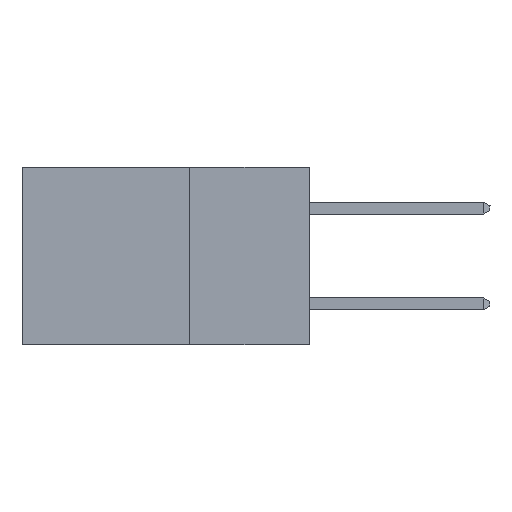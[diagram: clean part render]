
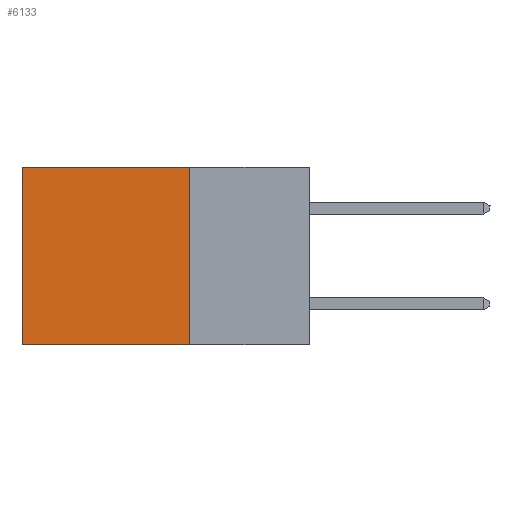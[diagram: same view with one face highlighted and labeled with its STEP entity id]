
A CAD part, left-side view. The second image highlights one B-rep face of the part: STEP entity #6133.
In plain terms, the highlighted planar face has unit normal (-1, 0, 0).
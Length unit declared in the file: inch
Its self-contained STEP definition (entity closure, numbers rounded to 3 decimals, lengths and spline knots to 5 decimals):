
#340 = ORIENTED_EDGE ( 'NONE', *, *, #2991, .F. ) ;
#1053 = AXIS2_PLACEMENT_3D ( 'NONE', #9230, #14562, #6903 ) ;
#1612 = LINE ( 'NONE', #5549, #1854 ) ;
#1854 = VECTOR ( 'NONE', #14796, 39.37008 ) ;
#2991 = EDGE_CURVE ( 'NONE', #8239, #18028, #9013, .T. ) ;
#3233 = EDGE_CURVE ( 'NONE', #5746, #12019, #11120, .T. ) ;
#5223 = CARTESIAN_POINT ( 'NONE',  ( 0.2875, 0.25, 0. ) ) ;
#5549 = CARTESIAN_POINT ( 'NONE',  ( 0.2875, 0.25, 0. ) ) ;
#5746 = VERTEX_POINT ( 'NONE', #5223 ) ;
#6041 = CARTESIAN_POINT ( 'NONE',  ( 0.2875, 0.25, -0.37 ) ) ;
#6133 = ADVANCED_FACE ( 'NONE', ( #7028 ), #20329, .F. ) ;
#6903 = DIRECTION ( 'NONE',  ( 0., 0., -1. ) ) ;
#7028 = FACE_OUTER_BOUND ( 'NONE', #16796, .T. ) ;
#7664 = DIRECTION ( 'NONE',  ( 0., 1., 0. ) ) ;
#7735 = CARTESIAN_POINT ( 'NONE',  ( 0.2875, 0.6, 0. ) ) ;
#8239 = VERTEX_POINT ( 'NONE', #6041 ) ;
#8493 = VECTOR ( 'NONE', #7664, 39.37008 ) ;
#9013 = LINE ( 'NONE', #16664, #9655 ) ;
#9230 = CARTESIAN_POINT ( 'NONE',  ( 0.2875, 0.25, 0. ) ) ;
#9655 = VECTOR ( 'NONE', #21806, 39.37008 ) ;
#11055 = ORIENTED_EDGE ( 'NONE', *, *, #14075, .T. ) ;
#11120 = LINE ( 'NONE', #18972, #8493 ) ;
#12019 = VERTEX_POINT ( 'NONE', #12813 ) ;
#12577 = CARTESIAN_POINT ( 'NONE',  ( 0.2875, 0.6, -0.37 ) ) ;
#12813 = CARTESIAN_POINT ( 'NONE',  ( 0.2875, 0.6, 0. ) ) ;
#14075 = EDGE_CURVE ( 'NONE', #12019, #18028, #15372, .T. ) ;
#14562 = DIRECTION ( 'NONE',  ( 1., 0., 0. ) ) ;
#14796 = DIRECTION ( 'NONE',  ( 0., 0., -1. ) ) ;
#15372 = LINE ( 'NONE', #7735, #18219 ) ;
#15550 = ORIENTED_EDGE ( 'NONE', *, *, #3233, .T. ) ;
#16664 = CARTESIAN_POINT ( 'NONE',  ( 0.2875, 0.25, -0.37 ) ) ;
#16796 = EDGE_LOOP ( 'NONE', ( #11055, #340, #19806, #15550 ) ) ;
#18028 = VERTEX_POINT ( 'NONE', #12577 ) ;
#18219 = VECTOR ( 'NONE', #22728, 39.37008 ) ;
#18972 = CARTESIAN_POINT ( 'NONE',  ( 0.2875, 0.25, 0. ) ) ;
#19806 = ORIENTED_EDGE ( 'NONE', *, *, #20264, .F. ) ;
#20264 = EDGE_CURVE ( 'NONE', #5746, #8239, #1612, .T. ) ;
#20329 = PLANE ( 'NONE',  #1053 ) ;
#21806 = DIRECTION ( 'NONE',  ( 0., 1., 0. ) ) ;
#22728 = DIRECTION ( 'NONE',  ( 0., 0., -1. ) ) ;
